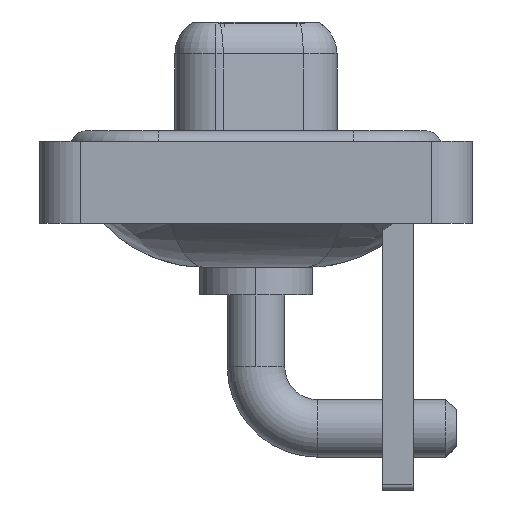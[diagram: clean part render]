
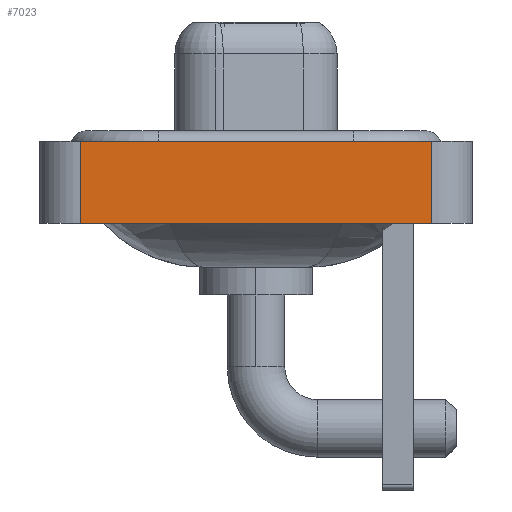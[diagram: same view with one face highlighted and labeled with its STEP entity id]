
A CAD part, left-side view. The second image highlights one B-rep face of the part: STEP entity #7023.
In plain terms, the highlighted planar face has unit normal (-1, 0, 0).
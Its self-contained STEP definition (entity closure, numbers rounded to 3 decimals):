
#138 = VERTEX_POINT ( 'NONE', #4609 ) ;
#947 = CARTESIAN_POINT ( 'NONE',  ( -7.35, -8.55, -3.6 ) ) ;
#1193 = LINE ( 'NONE', #10448, #15070 ) ;
#1251 = CARTESIAN_POINT ( 'NONE',  ( -7.35, -8.55, -3.6 ) ) ;
#1345 = CARTESIAN_POINT ( 'NONE',  ( -7.35, -8.55, 0.4 ) ) ;
#1692 = DIRECTION ( 'NONE',  ( 0., 0., 1. ) ) ;
#2463 = FACE_OUTER_BOUND ( 'NONE', #17141, .T. ) ;
#2519 = VERTEX_POINT ( 'NONE', #4200 ) ;
#3018 = EDGE_CURVE ( 'NONE', #13854, #5902, #1193, .T. ) ;
#3229 = VECTOR ( 'NONE', #11835, 1000. ) ;
#3846 = LINE ( 'NONE', #15765, #10257 ) ;
#4200 = CARTESIAN_POINT ( 'NONE',  ( -7.35, -8.55, 0.4 ) ) ;
#4297 = CARTESIAN_POINT ( 'NONE',  ( -7.35, -8.55, -3.6 ) ) ;
#4362 = DIRECTION ( 'NONE',  ( -1., 0., 0. ) ) ;
#4609 = CARTESIAN_POINT ( 'NONE',  ( -7.35, 8.55, 0.4 ) ) ;
#4703 = ORIENTED_EDGE ( 'NONE', *, *, #5498, .F. ) ;
#5498 = EDGE_CURVE ( 'NONE', #138, #2519, #6698, .T. ) ;
#5565 = AXIS2_PLACEMENT_3D ( 'NONE', #1251, #4362, #14367 ) ;
#5902 = VERTEX_POINT ( 'NONE', #947 ) ;
#6435 = VECTOR ( 'NONE', #1692, 1000. ) ;
#6698 = LINE ( 'NONE', #1345, #3229 ) ;
#7020 = ORIENTED_EDGE ( 'NONE', *, *, #15788, .F. ) ;
#7023 = ADVANCED_FACE ( 'NONE', ( #2463 ), #16359, .T. ) ;
#8650 = EDGE_CURVE ( 'NONE', #5902, #2519, #14884, .T. ) ;
#8988 = DIRECTION ( 'NONE',  ( 0., -1., 0. ) ) ;
#10169 = ORIENTED_EDGE ( 'NONE', *, *, #3018, .T. ) ;
#10254 = ORIENTED_EDGE ( 'NONE', *, *, #8650, .T. ) ;
#10257 = VECTOR ( 'NONE', #15683, 1000. ) ;
#10448 = CARTESIAN_POINT ( 'NONE',  ( -7.35, -8.55, -3.6 ) ) ;
#11659 = CARTESIAN_POINT ( 'NONE',  ( -7.35, 8.55, -3.6 ) ) ;
#11835 = DIRECTION ( 'NONE',  ( 0., -1., 0. ) ) ;
#13854 = VERTEX_POINT ( 'NONE', #11659 ) ;
#14367 = DIRECTION ( 'NONE',  ( 0., 0., 1. ) ) ;
#14884 = LINE ( 'NONE', #4297, #6435 ) ;
#15070 = VECTOR ( 'NONE', #8988, 1000. ) ;
#15683 = DIRECTION ( 'NONE',  ( 0., 0., 1. ) ) ;
#15765 = CARTESIAN_POINT ( 'NONE',  ( -7.35, 8.55, -3.6 ) ) ;
#15788 = EDGE_CURVE ( 'NONE', #13854, #138, #3846, .T. ) ;
#16359 = PLANE ( 'NONE',  #5565 ) ;
#17141 = EDGE_LOOP ( 'NONE', ( #10254, #4703, #7020, #10169 ) ) ;
